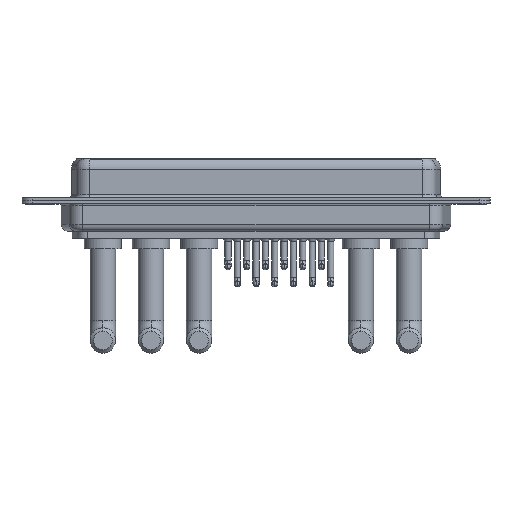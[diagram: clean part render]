
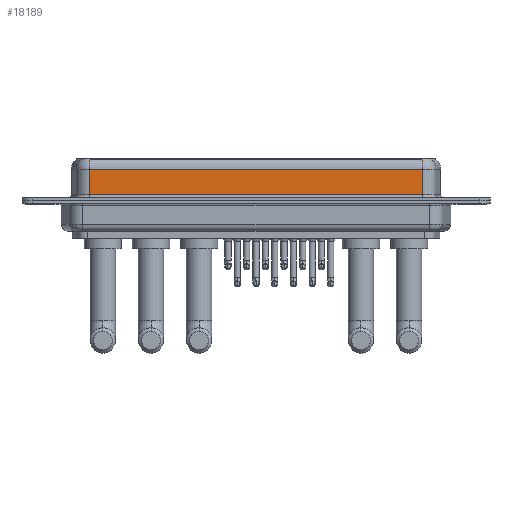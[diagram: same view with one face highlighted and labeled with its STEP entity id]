
A CAD part, front view. The second image highlights one B-rep face of the part: STEP entity #18189.
In plain terms, the highlighted planar face has unit normal (0, -1, 0).
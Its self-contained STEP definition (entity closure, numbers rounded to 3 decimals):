
#729 = VECTOR ( 'NONE', #12317, 1000. ) ;
#851 = ORIENTED_EDGE ( 'NONE', *, *, #10406, .T. ) ;
#1100 = VERTEX_POINT ( 'NONE', #9493 ) ;
#2174 = EDGE_LOOP ( 'NONE', ( #2958, #6836, #16588, #851 ) ) ;
#2955 = VERTEX_POINT ( 'NONE', #7158 ) ;
#2958 = ORIENTED_EDGE ( 'NONE', *, *, #4507, .F. ) ;
#3143 = EDGE_CURVE ( 'NONE', #2955, #17763, #14122, .T. ) ;
#3636 = DIRECTION ( 'NONE',  ( 0., 1., 0. ) ) ;
#3732 = CARTESIAN_POINT ( 'NONE',  ( 56.462, -3.95, 0.9 ) ) ;
#4507 = EDGE_CURVE ( 'NONE', #2955, #1100, #16401, .T. ) ;
#5171 = CARTESIAN_POINT ( 'NONE',  ( 56.462, -3.95, 4.65 ) ) ;
#5646 = VECTOR ( 'NONE', #12206, 1000. ) ;
#6530 = CARTESIAN_POINT ( 'NONE',  ( 56.462, -3.95, 6.4 ) ) ;
#6836 = ORIENTED_EDGE ( 'NONE', *, *, #3143, .T. ) ;
#6968 = CARTESIAN_POINT ( 'NONE',  ( 7.038, -3.95, 4.65 ) ) ;
#7120 = DIRECTION ( 'NONE',  ( 0., 0., 1. ) ) ;
#7158 = CARTESIAN_POINT ( 'NONE',  ( 56.462, -3.95, 4.65 ) ) ;
#9493 = CARTESIAN_POINT ( 'NONE',  ( 56.462, -3.95, 0.9 ) ) ;
#9938 = LINE ( 'NONE', #14316, #15140 ) ;
#10406 = EDGE_CURVE ( 'NONE', #11587, #1100, #17897, .T. ) ;
#11325 = DIRECTION ( 'NONE',  ( 0., 0., -1. ) ) ;
#11587 = VERTEX_POINT ( 'NONE', #12134 ) ;
#12134 = CARTESIAN_POINT ( 'NONE',  ( 7.038, -3.95, 0.9 ) ) ;
#12206 = DIRECTION ( 'NONE',  ( 0., 0., -1. ) ) ;
#12317 = DIRECTION ( 'NONE',  ( 1., 0., 0. ) ) ;
#12533 = DIRECTION ( 'NONE',  ( -1., 0., 0. ) ) ;
#12694 = PLANE ( 'NONE',  #17532 ) ;
#13358 = VECTOR ( 'NONE', #12533, 1000. ) ;
#14122 = LINE ( 'NONE', #5171, #13358 ) ;
#14316 = CARTESIAN_POINT ( 'NONE',  ( 7.038, -3.95, 6.4 ) ) ;
#15140 = VECTOR ( 'NONE', #11325, 1000. ) ;
#15401 = FACE_OUTER_BOUND ( 'NONE', #2174, .T. ) ;
#16401 = LINE ( 'NONE', #6530, #5646 ) ;
#16588 = ORIENTED_EDGE ( 'NONE', *, *, #17245, .T. ) ;
#17245 = EDGE_CURVE ( 'NONE', #17763, #11587, #9938, .T. ) ;
#17532 = AXIS2_PLACEMENT_3D ( 'NONE', #18373, #3636, #7120 ) ;
#17763 = VERTEX_POINT ( 'NONE', #6968 ) ;
#17897 = LINE ( 'NONE', #3732, #729 ) ;
#18189 = ADVANCED_FACE ( 'NONE', ( #15401 ), #12694, .F. ) ;
#18373 = CARTESIAN_POINT ( 'NONE',  ( 56.462, -3.95, 6.4 ) ) ;
